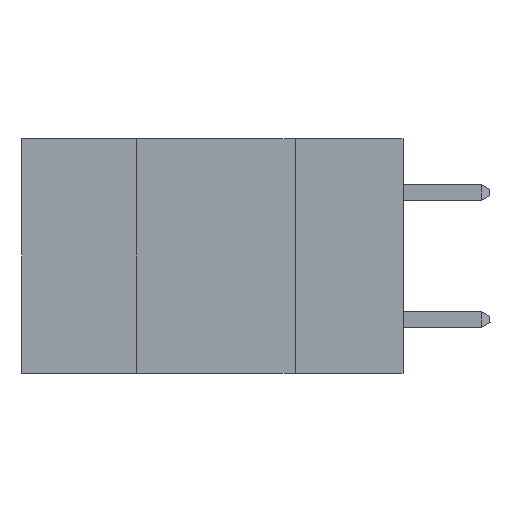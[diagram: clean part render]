
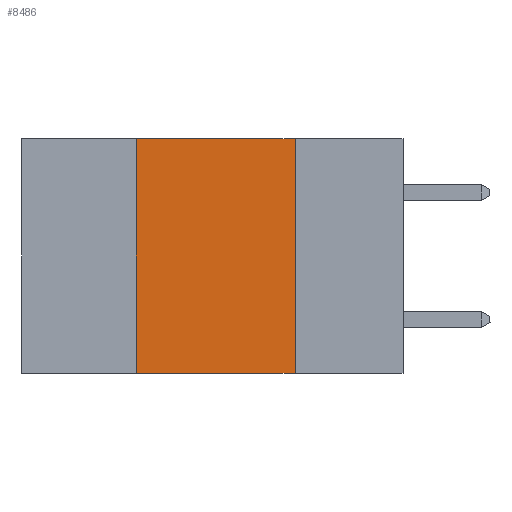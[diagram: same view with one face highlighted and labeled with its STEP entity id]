
A CAD part, left-side view. The second image highlights one B-rep face of the part: STEP entity #8486.
In plain terms, the highlighted planar face has unit normal (-1, 0, 0).
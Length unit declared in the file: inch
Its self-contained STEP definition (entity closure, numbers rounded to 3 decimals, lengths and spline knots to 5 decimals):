
#102 = CARTESIAN_POINT ( 'NONE',  ( 0., 0.42, 0. ) ) ;
#145 = VECTOR ( 'NONE', #2703, 39.37008 ) ;
#879 = CARTESIAN_POINT ( 'NONE',  ( 0., 0.6, 0. ) ) ;
#923 = DIRECTION ( 'NONE',  ( 0., -1., 0. ) ) ;
#1896 = EDGE_LOOP ( 'NONE', ( #7148, #7465, #12105, #2031 ) ) ;
#1915 = DIRECTION ( 'NONE',  ( 1., 0., 0. ) ) ;
#2031 = ORIENTED_EDGE ( 'NONE', *, *, #7698, .T. ) ;
#2078 = EDGE_CURVE ( 'NONE', #6092, #5918, #6932, .T. ) ;
#2411 = EDGE_CURVE ( 'NONE', #6382, #2646, #10798, .T. ) ;
#2646 = VERTEX_POINT ( 'NONE', #102 ) ;
#2703 = DIRECTION ( 'NONE',  ( 0., 0., 1. ) ) ;
#2932 = LINE ( 'NONE', #7618, #12156 ) ;
#3812 = DIRECTION ( 'NONE',  ( 0., -1., 0. ) ) ;
#4134 = CARTESIAN_POINT ( 'NONE',  ( 0., 0.17, -0.37 ) ) ;
#5120 = DIRECTION ( 'NONE',  ( 0., 0., -1. ) ) ;
#5631 = CARTESIAN_POINT ( 'NONE',  ( 0., 0.42, 0. ) ) ;
#5918 = VERTEX_POINT ( 'NONE', #4134 ) ;
#6092 = VERTEX_POINT ( 'NONE', #10159 ) ;
#6342 = EDGE_CURVE ( 'NONE', #2646, #6092, #9930, .T. ) ;
#6382 = VERTEX_POINT ( 'NONE', #9843 ) ;
#6932 = LINE ( 'NONE', #9731, #9099 ) ;
#7098 = AXIS2_PLACEMENT_3D ( 'NONE', #12172, #1915, #8716 ) ;
#7148 = ORIENTED_EDGE ( 'NONE', *, *, #2078, .F. ) ;
#7465 = ORIENTED_EDGE ( 'NONE', *, *, #6342, .F. ) ;
#7618 = CARTESIAN_POINT ( 'NONE',  ( 0., 0.6, -0.37 ) ) ;
#7698 = EDGE_CURVE ( 'NONE', #6382, #5918, #2932, .T. ) ;
#8486 = ADVANCED_FACE ( 'NONE', ( #11401 ), #11356, .F. ) ;
#8716 = DIRECTION ( 'NONE',  ( 0., 0., -1. ) ) ;
#9099 = VECTOR ( 'NONE', #5120, 39.37008 ) ;
#9731 = CARTESIAN_POINT ( 'NONE',  ( 0., 0.17, 0. ) ) ;
#9843 = CARTESIAN_POINT ( 'NONE',  ( 0., 0.42, -0.37 ) ) ;
#9930 = LINE ( 'NONE', #879, #10208 ) ;
#10159 = CARTESIAN_POINT ( 'NONE',  ( 0., 0.17, 0. ) ) ;
#10208 = VECTOR ( 'NONE', #923, 39.37008 ) ;
#10798 = LINE ( 'NONE', #5631, #145 ) ;
#11356 = PLANE ( 'NONE',  #7098 ) ;
#11401 = FACE_OUTER_BOUND ( 'NONE', #1896, .T. ) ;
#12105 = ORIENTED_EDGE ( 'NONE', *, *, #2411, .F. ) ;
#12156 = VECTOR ( 'NONE', #3812, 39.37008 ) ;
#12172 = CARTESIAN_POINT ( 'NONE',  ( 0., 0.6, 0. ) ) ;
